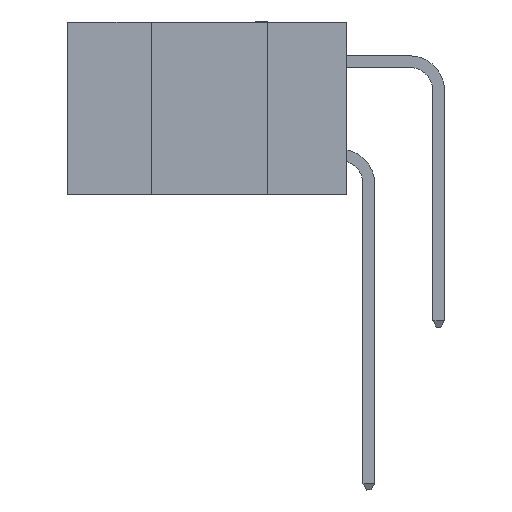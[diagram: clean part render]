
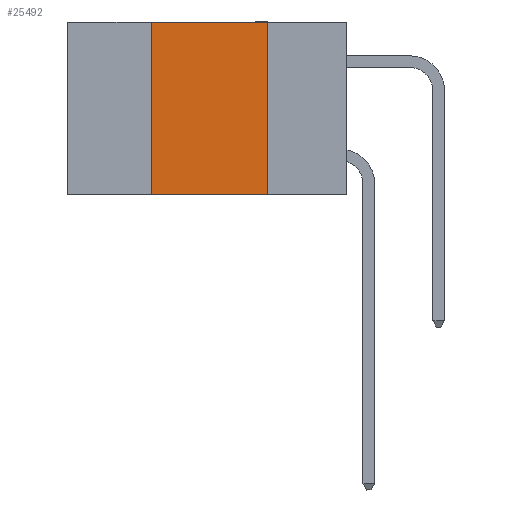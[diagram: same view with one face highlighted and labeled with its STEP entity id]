
A CAD part, left-side view. The second image highlights one B-rep face of the part: STEP entity #25492.
In plain terms, the highlighted planar face has unit normal (-1, 0, 0).
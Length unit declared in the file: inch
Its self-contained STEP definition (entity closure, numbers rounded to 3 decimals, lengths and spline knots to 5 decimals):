
#275 = CARTESIAN_POINT ( 'NONE',  ( 0., 0.42, -0.37 ) ) ;
#1143 = EDGE_CURVE ( 'NONE', #19059, #26907, #18533, .T. ) ;
#3005 = LINE ( 'NONE', #3130, #21244 ) ;
#3130 = CARTESIAN_POINT ( 'NONE',  ( 0., 0.6, 0. ) ) ;
#4156 = EDGE_CURVE ( 'NONE', #19059, #13491, #17582, .T. ) ;
#4669 = CARTESIAN_POINT ( 'NONE',  ( 0., 0.42, 0. ) ) ;
#4887 = DIRECTION ( 'NONE',  ( 0., 0., 1. ) ) ;
#6207 = EDGE_LOOP ( 'NONE', ( #27639, #27398, #22827, #10704 ) ) ;
#10040 = CARTESIAN_POINT ( 'NONE',  ( 0., 0.17, 0. ) ) ;
#10138 = DIRECTION ( 'NONE',  ( 1., 0., 0. ) ) ;
#10310 = CARTESIAN_POINT ( 'NONE',  ( 0., 0.42, 0. ) ) ;
#10704 = ORIENTED_EDGE ( 'NONE', *, *, #4156, .T. ) ;
#12605 = DIRECTION ( 'NONE',  ( 0., 0., -1. ) ) ;
#13476 = EDGE_CURVE ( 'NONE', #21871, #13491, #17726, .T. ) ;
#13491 = VERTEX_POINT ( 'NONE', #19686 ) ;
#14469 = CARTESIAN_POINT ( 'NONE',  ( 0., 0.17, 0. ) ) ;
#14479 = DIRECTION ( 'NONE',  ( 0., -1., 0. ) ) ;
#15711 = VECTOR ( 'NONE', #14479, 39.37008 ) ;
#15951 = AXIS2_PLACEMENT_3D ( 'NONE', #26714, #10138, #19256 ) ;
#17099 = CARTESIAN_POINT ( 'NONE',  ( 0., 0.6, -0.37 ) ) ;
#17282 = EDGE_CURVE ( 'NONE', #26907, #21871, #3005, .T. ) ;
#17582 = LINE ( 'NONE', #17099, #15711 ) ;
#17726 = LINE ( 'NONE', #10040, #18472 ) ;
#18472 = VECTOR ( 'NONE', #12605, 39.37008 ) ;
#18533 = LINE ( 'NONE', #4669, #29391 ) ;
#19059 = VERTEX_POINT ( 'NONE', #275 ) ;
#19256 = DIRECTION ( 'NONE',  ( 0., 0., -1. ) ) ;
#19686 = CARTESIAN_POINT ( 'NONE',  ( 0., 0.17, -0.37 ) ) ;
#19774 = DIRECTION ( 'NONE',  ( 0., -1., 0. ) ) ;
#21244 = VECTOR ( 'NONE', #19774, 39.37008 ) ;
#21871 = VERTEX_POINT ( 'NONE', #14469 ) ;
#22827 = ORIENTED_EDGE ( 'NONE', *, *, #1143, .F. ) ;
#23980 = PLANE ( 'NONE',  #15951 ) ;
#25492 = ADVANCED_FACE ( 'NONE', ( #25744 ), #23980, .F. ) ;
#25744 = FACE_OUTER_BOUND ( 'NONE', #6207, .T. ) ;
#26714 = CARTESIAN_POINT ( 'NONE',  ( 0., 0.6, 0. ) ) ;
#26907 = VERTEX_POINT ( 'NONE', #10310 ) ;
#27398 = ORIENTED_EDGE ( 'NONE', *, *, #17282, .F. ) ;
#27639 = ORIENTED_EDGE ( 'NONE', *, *, #13476, .F. ) ;
#29391 = VECTOR ( 'NONE', #4887, 39.37008 ) ;
